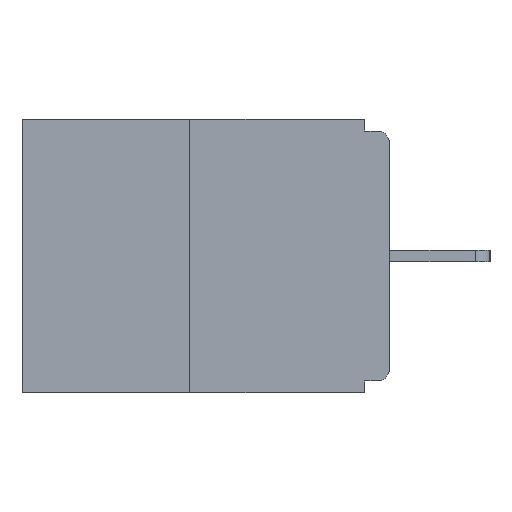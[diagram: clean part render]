
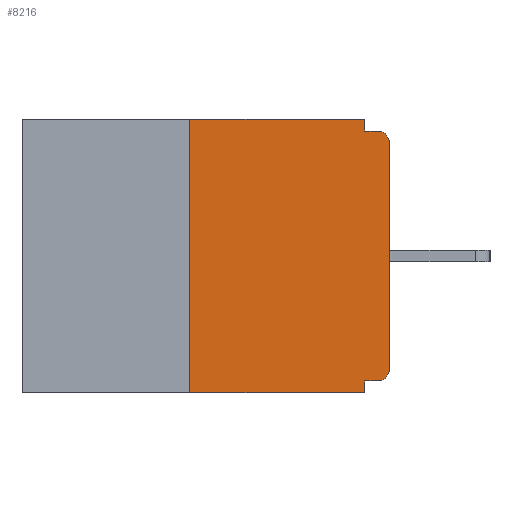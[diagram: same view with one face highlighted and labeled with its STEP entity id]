
A CAD part, left-side view. The second image highlights one B-rep face of the part: STEP entity #8216.
In plain terms, the highlighted planar face has unit normal (-1, 0, 0).
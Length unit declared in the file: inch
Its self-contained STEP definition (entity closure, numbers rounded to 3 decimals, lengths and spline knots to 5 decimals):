
#300 = LINE ( 'NONE', #12658, #5841 ) ;
#303 = VERTEX_POINT ( 'NONE', #2471 ) ;
#358 = LINE ( 'NONE', #12460, #5880 ) ;
#490 = VERTEX_POINT ( 'NONE', #3460 ) ;
#618 = VECTOR ( 'NONE', #7090, 39.37008 ) ;
#661 = DIRECTION ( 'NONE',  ( 0., 0., -1. ) ) ;
#900 = ORIENTED_EDGE ( 'NONE', *, *, #9646, .F. ) ;
#1023 = AXIS2_PLACEMENT_3D ( 'NONE', #12423, #6336, #2716 ) ;
#1041 = ORIENTED_EDGE ( 'NONE', *, *, #9888, .T. ) ;
#1475 = DIRECTION ( 'NONE',  ( 0., 0., -1. ) ) ;
#1576 = VECTOR ( 'NONE', #4897, 39.37008 ) ;
#1704 = ORIENTED_EDGE ( 'NONE', *, *, #10469, .F. ) ;
#1836 = VERTEX_POINT ( 'NONE', #8215 ) ;
#2471 = CARTESIAN_POINT ( 'NONE',  ( 0., 0.25, -0.343 ) ) ;
#2716 = DIRECTION ( 'NONE',  ( 0., 0., -1. ) ) ;
#2784 = ORIENTED_EDGE ( 'NONE', *, *, #10518, .F. ) ;
#2793 = DIRECTION ( 'NONE',  ( 0., 0., 1. ) ) ;
#2812 = CARTESIAN_POINT ( 'NONE',  ( 0., 0.015, -0.015 ) ) ;
#2874 = EDGE_CURVE ( 'NONE', #303, #6723, #15425, .T. ) ;
#3141 = VERTEX_POINT ( 'NONE', #13803 ) ;
#3209 = CARTESIAN_POINT ( 'NONE',  ( 0., 0.031, -0.343 ) ) ;
#3460 = CARTESIAN_POINT ( 'NONE',  ( 0., 0.25, 0. ) ) ;
#3698 = VECTOR ( 'NONE', #6611, 39.37008 ) ;
#3734 = LINE ( 'NONE', #13453, #13017 ) ;
#3777 = CARTESIAN_POINT ( 'NONE',  ( 0., 0., -0.328 ) ) ;
#4045 = CARTESIAN_POINT ( 'NONE',  ( 0., 0., -0.313 ) ) ;
#4387 = VERTEX_POINT ( 'NONE', #2812 ) ;
#4627 = CIRCLE ( 'NONE', #5143, 0.015 ) ;
#4897 = DIRECTION ( 'NONE',  ( 0., -1., 0. ) ) ;
#4968 = CARTESIAN_POINT ( 'NONE',  ( 0., 0.46, 0. ) ) ;
#5018 = DIRECTION ( 'NONE',  ( 0., 0., -1. ) ) ;
#5043 = LINE ( 'NONE', #4968, #1576 ) ;
#5143 = AXIS2_PLACEMENT_3D ( 'NONE', #13238, #9550, #15550 ) ;
#5145 = ORIENTED_EDGE ( 'NONE', *, *, #14826, .F. ) ;
#5156 = LINE ( 'NONE', #3777, #11533 ) ;
#5841 = VECTOR ( 'NONE', #15148, 39.37008 ) ;
#5880 = VECTOR ( 'NONE', #1475, 39.37008 ) ;
#6203 = EDGE_LOOP ( 'NONE', ( #900, #7783, #7267, #5145, #1704, #15746, #7345, #1041, #8834, #2784 ) ) ;
#6315 = EDGE_CURVE ( 'NONE', #3141, #4387, #9575, .T. ) ;
#6336 = DIRECTION ( 'NONE',  ( 1., 0., 0. ) ) ;
#6611 = DIRECTION ( 'NONE',  ( 0., -1., 0. ) ) ;
#6614 = DIRECTION ( 'NONE',  ( 0., 1., 0. ) ) ;
#6723 = VERTEX_POINT ( 'NONE', #3209 ) ;
#7090 = DIRECTION ( 'NONE',  ( 0., -1., 0. ) ) ;
#7104 = VERTEX_POINT ( 'NONE', #15394 ) ;
#7267 = ORIENTED_EDGE ( 'NONE', *, *, #2874, .T. ) ;
#7345 = ORIENTED_EDGE ( 'NONE', *, *, #12641, .T. ) ;
#7397 = VERTEX_POINT ( 'NONE', #7448 ) ;
#7448 = CARTESIAN_POINT ( 'NONE',  ( 0., 0.031, -0.328 ) ) ;
#7547 = PLANE ( 'NONE',  #1023 ) ;
#7683 = AXIS2_PLACEMENT_3D ( 'NONE', #13164, #14437, #661 ) ;
#7783 = ORIENTED_EDGE ( 'NONE', *, *, #15027, .F. ) ;
#7971 = EDGE_CURVE ( 'NONE', #7104, #15506, #11503, .T. ) ;
#8099 = CARTESIAN_POINT ( 'NONE',  ( 0., 0., -0.03 ) ) ;
#8147 = CARTESIAN_POINT ( 'NONE',  ( 0., 0., -0.015 ) ) ;
#8215 = CARTESIAN_POINT ( 'NONE',  ( 0., 0.031, 0. ) ) ;
#8216 = ADVANCED_FACE ( 'NONE', ( #10344 ), #7547, .F. ) ;
#8834 = ORIENTED_EDGE ( 'NONE', *, *, #6315, .F. ) ;
#9550 = DIRECTION ( 'NONE',  ( -1., 0., 0. ) ) ;
#9575 = LINE ( 'NONE', #8147, #618 ) ;
#9646 = EDGE_CURVE ( 'NONE', #490, #1836, #5043, .T. ) ;
#9888 = EDGE_CURVE ( 'NONE', #11518, #4387, #4627, .T. ) ;
#10344 = FACE_OUTER_BOUND ( 'NONE', #6203, .T. ) ;
#10469 = EDGE_CURVE ( 'NONE', #7104, #7397, #5156, .T. ) ;
#10518 = EDGE_CURVE ( 'NONE', #1836, #3141, #358, .T. ) ;
#11503 = CIRCLE ( 'NONE', #7683, 0.015 ) ;
#11518 = VERTEX_POINT ( 'NONE', #8099 ) ;
#11533 = VECTOR ( 'NONE', #6614, 39.37008 ) ;
#12423 = CARTESIAN_POINT ( 'NONE',  ( 0., 0.46, 0. ) ) ;
#12460 = CARTESIAN_POINT ( 'NONE',  ( 0., 0.031, 0. ) ) ;
#12641 = EDGE_CURVE ( 'NONE', #15506, #11518, #13539, .T. ) ;
#12658 = CARTESIAN_POINT ( 'NONE',  ( 0., 0.25, 0. ) ) ;
#13017 = VECTOR ( 'NONE', #5018, 39.37008 ) ;
#13164 = CARTESIAN_POINT ( 'NONE',  ( 0., 0.015, -0.313 ) ) ;
#13238 = CARTESIAN_POINT ( 'NONE',  ( 0., 0.015, -0.03 ) ) ;
#13453 = CARTESIAN_POINT ( 'NONE',  ( 0., 0.031, -0.343 ) ) ;
#13539 = LINE ( 'NONE', #14743, #13997 ) ;
#13803 = CARTESIAN_POINT ( 'NONE',  ( 0., 0.031, -0.015 ) ) ;
#13997 = VECTOR ( 'NONE', #2793, 39.37008 ) ;
#14437 = DIRECTION ( 'NONE',  ( -1., 0., 0. ) ) ;
#14743 = CARTESIAN_POINT ( 'NONE',  ( 0., 0., 0. ) ) ;
#14826 = EDGE_CURVE ( 'NONE', #7397, #6723, #3734, .T. ) ;
#15027 = EDGE_CURVE ( 'NONE', #303, #490, #300, .T. ) ;
#15148 = DIRECTION ( 'NONE',  ( 0., 0., 1. ) ) ;
#15349 = CARTESIAN_POINT ( 'NONE',  ( 0., 0.46, -0.343 ) ) ;
#15394 = CARTESIAN_POINT ( 'NONE',  ( 0., 0.015, -0.328 ) ) ;
#15425 = LINE ( 'NONE', #15349, #3698 ) ;
#15506 = VERTEX_POINT ( 'NONE', #4045 ) ;
#15550 = DIRECTION ( 'NONE',  ( 0., 0., -1. ) ) ;
#15746 = ORIENTED_EDGE ( 'NONE', *, *, #7971, .T. ) ;
